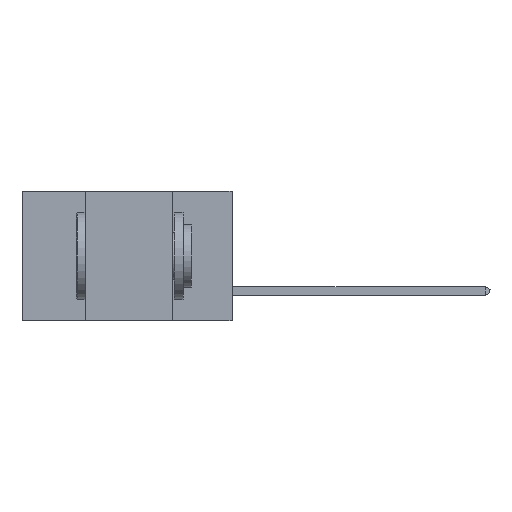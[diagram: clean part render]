
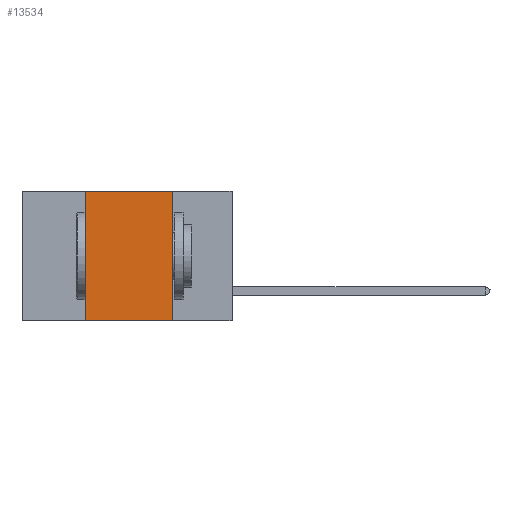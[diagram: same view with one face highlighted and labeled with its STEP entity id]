
A CAD part, left-side view. The second image highlights one B-rep face of the part: STEP entity #13534.
In plain terms, the highlighted planar face has unit normal (-1, 0, 0).
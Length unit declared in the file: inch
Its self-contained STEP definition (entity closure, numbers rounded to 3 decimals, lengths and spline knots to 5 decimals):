
#885 = FACE_OUTER_BOUND ( 'NONE', #10414, .T. ) ;
#1160 = CARTESIAN_POINT ( 'NONE',  ( 0., 0.42, -0.37 ) ) ;
#2037 = ORIENTED_EDGE ( 'NONE', *, *, #14945, .F. ) ;
#2291 = VERTEX_POINT ( 'NONE', #1160 ) ;
#3330 = EDGE_CURVE ( 'NONE', #2291, #5735, #4512, .T. ) ;
#4512 = LINE ( 'NONE', #21517, #5539 ) ;
#4809 = ORIENTED_EDGE ( 'NONE', *, *, #3330, .T. ) ;
#5039 = DIRECTION ( 'NONE',  ( 1., 0., 0. ) ) ;
#5539 = VECTOR ( 'NONE', #9530, 39.37008 ) ;
#5735 = VERTEX_POINT ( 'NONE', #7449 ) ;
#5917 = CARTESIAN_POINT ( 'NONE',  ( 0., 0.42, 0. ) ) ;
#6315 = CARTESIAN_POINT ( 'NONE',  ( 0., 0.42, 0. ) ) ;
#7449 = CARTESIAN_POINT ( 'NONE',  ( 0., 0.17, -0.37 ) ) ;
#8260 = DIRECTION ( 'NONE',  ( 0., 0., -1. ) ) ;
#9068 = DIRECTION ( 'NONE',  ( 0., 0., -1. ) ) ;
#9133 = CARTESIAN_POINT ( 'NONE',  ( 0., 0.17, 0. ) ) ;
#9530 = DIRECTION ( 'NONE',  ( 0., -1., 0. ) ) ;
#9623 = VECTOR ( 'NONE', #9068, 39.37008 ) ;
#10013 = LINE ( 'NONE', #12865, #18360 ) ;
#10414 = EDGE_LOOP ( 'NONE', ( #19485, #18731, #2037, #4809 ) ) ;
#12346 = LINE ( 'NONE', #5917, #17522 ) ;
#12530 = VERTEX_POINT ( 'NONE', #6315 ) ;
#12786 = LINE ( 'NONE', #9133, #9623 ) ;
#12865 = CARTESIAN_POINT ( 'NONE',  ( 0., 0.6, 0. ) ) ;
#13417 = EDGE_CURVE ( 'NONE', #12530, #19825, #10013, .T. ) ;
#13534 = ADVANCED_FACE ( 'NONE', ( #885 ), #15046, .F. ) ;
#14282 = AXIS2_PLACEMENT_3D ( 'NONE', #14901, #5039, #8260 ) ;
#14676 = DIRECTION ( 'NONE',  ( 0., -1., 0. ) ) ;
#14901 = CARTESIAN_POINT ( 'NONE',  ( 0., 0.6, 0. ) ) ;
#14945 = EDGE_CURVE ( 'NONE', #2291, #12530, #12346, .T. ) ;
#15046 = PLANE ( 'NONE',  #14282 ) ;
#16730 = EDGE_CURVE ( 'NONE', #19825, #5735, #12786, .T. ) ;
#17522 = VECTOR ( 'NONE', #20893, 39.37008 ) ;
#18360 = VECTOR ( 'NONE', #14676, 39.37008 ) ;
#18403 = CARTESIAN_POINT ( 'NONE',  ( 0., 0.17, 0. ) ) ;
#18731 = ORIENTED_EDGE ( 'NONE', *, *, #13417, .F. ) ;
#19485 = ORIENTED_EDGE ( 'NONE', *, *, #16730, .F. ) ;
#19825 = VERTEX_POINT ( 'NONE', #18403 ) ;
#20893 = DIRECTION ( 'NONE',  ( 0., 0., 1. ) ) ;
#21517 = CARTESIAN_POINT ( 'NONE',  ( 0., 0.6, -0.37 ) ) ;
